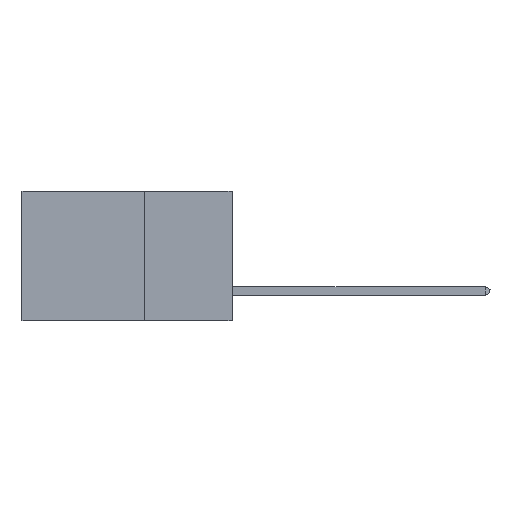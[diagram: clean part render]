
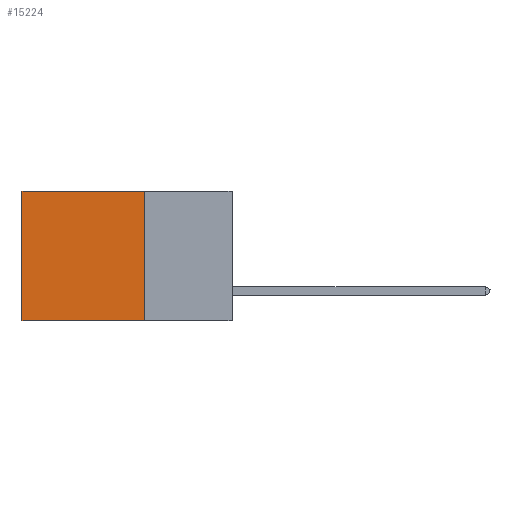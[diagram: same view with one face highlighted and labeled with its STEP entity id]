
A CAD part, left-side view. The second image highlights one B-rep face of the part: STEP entity #15224.
In plain terms, the highlighted planar face has unit normal (-1, 0, 0).
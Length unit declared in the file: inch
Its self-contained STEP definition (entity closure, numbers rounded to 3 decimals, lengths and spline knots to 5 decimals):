
#826 = DIRECTION ( 'NONE',  ( 0., 0., -1. ) ) ;
#1163 = CARTESIAN_POINT ( 'NONE',  ( 0.2875, 0.6, -0.37 ) ) ;
#1525 = LINE ( 'NONE', #18609, #13523 ) ;
#1923 = CARTESIAN_POINT ( 'NONE',  ( 0.2875, 0.6, 0. ) ) ;
#2130 = CARTESIAN_POINT ( 'NONE',  ( 0.2875, 0.25, 0. ) ) ;
#2210 = EDGE_CURVE ( 'NONE', #13356, #11838, #16842, .T. ) ;
#2891 = DIRECTION ( 'NONE',  ( 0., 1., 0. ) ) ;
#3230 = VECTOR ( 'NONE', #2891, 39.37008 ) ;
#3831 = LINE ( 'NONE', #2130, #17168 ) ;
#4065 = EDGE_CURVE ( 'NONE', #15143, #11838, #1525, .T. ) ;
#4289 = ORIENTED_EDGE ( 'NONE', *, *, #8490, .T. ) ;
#5590 = ORIENTED_EDGE ( 'NONE', *, *, #4065, .T. ) ;
#6049 = DIRECTION ( 'NONE',  ( 0., 0., -1. ) ) ;
#6114 = CARTESIAN_POINT ( 'NONE',  ( 0.2875, 0.25, 0. ) ) ;
#6610 = DIRECTION ( 'NONE',  ( 1., 0., 0. ) ) ;
#6823 = VERTEX_POINT ( 'NONE', #11126 ) ;
#7071 = AXIS2_PLACEMENT_3D ( 'NONE', #8089, #6610, #826 ) ;
#7458 = EDGE_CURVE ( 'NONE', #6823, #13356, #15607, .T. ) ;
#7732 = VECTOR ( 'NONE', #6049, 39.37008 ) ;
#8089 = CARTESIAN_POINT ( 'NONE',  ( 0.2875, 0.25, 0. ) ) ;
#8429 = ORIENTED_EDGE ( 'NONE', *, *, #7458, .F. ) ;
#8490 = EDGE_CURVE ( 'NONE', #6823, #15143, #3831, .T. ) ;
#8713 = CARTESIAN_POINT ( 'NONE',  ( 0.2875, 0.25, -0.37 ) ) ;
#9397 = ORIENTED_EDGE ( 'NONE', *, *, #2210, .F. ) ;
#9431 = DIRECTION ( 'NONE',  ( 0., 1., 0. ) ) ;
#9585 = DIRECTION ( 'NONE',  ( 0., 0., -1. ) ) ;
#11023 = PLANE ( 'NONE',  #7071 ) ;
#11126 = CARTESIAN_POINT ( 'NONE',  ( 0.2875, 0.25, 0. ) ) ;
#11608 = CARTESIAN_POINT ( 'NONE',  ( 0.2875, 0.25, -0.37 ) ) ;
#11718 = EDGE_LOOP ( 'NONE', ( #5590, #9397, #8429, #4289 ) ) ;
#11838 = VERTEX_POINT ( 'NONE', #1163 ) ;
#13356 = VERTEX_POINT ( 'NONE', #11608 ) ;
#13523 = VECTOR ( 'NONE', #9585, 39.37008 ) ;
#14344 = FACE_OUTER_BOUND ( 'NONE', #11718, .T. ) ;
#15143 = VERTEX_POINT ( 'NONE', #1923 ) ;
#15224 = ADVANCED_FACE ( 'NONE', ( #14344 ), #11023, .F. ) ;
#15607 = LINE ( 'NONE', #6114, #7732 ) ;
#16842 = LINE ( 'NONE', #8713, #3230 ) ;
#17168 = VECTOR ( 'NONE', #9431, 39.37008 ) ;
#18609 = CARTESIAN_POINT ( 'NONE',  ( 0.2875, 0.6, 0. ) ) ;
